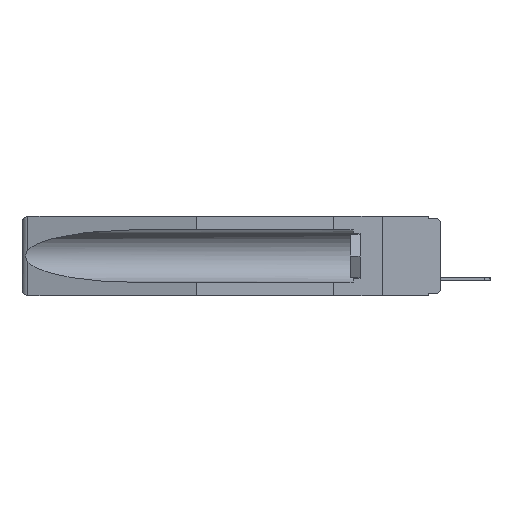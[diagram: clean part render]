
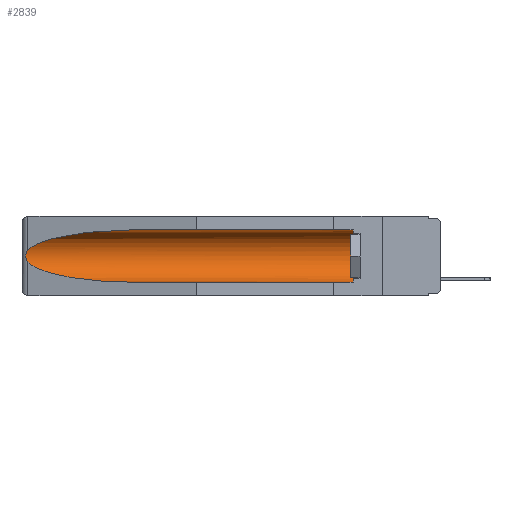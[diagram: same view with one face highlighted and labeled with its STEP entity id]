
A CAD part, left-side view. The second image highlights one B-rep face of the part: STEP entity #2839.
In plain terms, the highlighted cylindrical face has radius 2.857 mm (diameter 5.715 mm), a partial arc.
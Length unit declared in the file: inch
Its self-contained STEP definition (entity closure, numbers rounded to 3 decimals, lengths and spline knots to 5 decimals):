
#950 = CARTESIAN_POINT ( 'NONE',  ( 0.26537, 1.52718, -0.19328 ) ) ;
#1172 = DIRECTION ( 'NONE',  ( 0., 0., 1. ) ) ;
#1222 = CARTESIAN_POINT ( 'NONE',  ( 0.155, 0.126, -0.059 ) ) ;
#1223 = VERTEX_POINT ( 'NONE', #7573 ) ;
#1443 = CARTESIAN_POINT ( 'NONE',  ( 0.21114, 1.30732, -0.059 ) ) ;
#2048 = DIRECTION ( 'NONE',  ( 0., 1., 0. ) ) ;
#2408 = CARTESIAN_POINT ( 'NONE',  ( 0.21114, 1.30732, -0.284 ) ) ;
#2552 = CARTESIAN_POINT ( 'NONE',  ( 0.25451, 1.48313, -0.24835 ) ) ;
#2839 = ADVANCED_FACE ( 'NONE', ( #8455 ), #10889, .F. ) ;
#3240 = CARTESIAN_POINT ( 'NONE',  ( 0.26537, 1.52718, -0.14972 ) ) ;
#3303 = CARTESIAN_POINT ( 'NONE',  ( 0.155, 1.07973, -0.059 ) ) ;
#3367 = CIRCLE ( 'NONE', #21112, 0.1125 ) ;
#3455 = ORIENTED_EDGE ( 'NONE', *, *, #9971, .F. ) ;
#3462 =( BOUNDED_CURVE ( )  B_SPLINE_CURVE ( 3, ( #3303, #1443, #12286, #3732 ),
 .UNSPECIFIED., .F., .T. ) 
 B_SPLINE_CURVE_WITH_KNOTS ( ( 4, 4 ),
 ( 4.71239, 6.08839 ),
 .UNSPECIFIED. ) 
 CURVE ( )  GEOMETRIC_REPRESENTATION_ITEM ( )  RATIONAL_B_SPLINE_CURVE ( ( 1., 0.848, 0.848, 1. ) ) 
 REPRESENTATION_ITEM ( '' )  );
#3666 = CARTESIAN_POINT ( 'NONE',  ( 0.26655, 1.53094, -0.18657 ) ) ;
#3732 = CARTESIAN_POINT ( 'NONE',  ( 0.26537, 1.52718, -0.14972 ) ) ;
#3931 = CARTESIAN_POINT ( 'NONE',  ( 0.155, -0.30754, -0.284 ) ) ;
#5102 = VERTEX_POINT ( 'NONE', #9609 ) ;
#5926 = CARTESIAN_POINT ( 'NONE',  ( 0.26537, 1.52718, -0.19328 ) ) ;
#7573 = CARTESIAN_POINT ( 'NONE',  ( 0.26537, 1.52718, -0.14972 ) ) ;
#7783 = CARTESIAN_POINT ( 'NONE',  ( 0.26597, 1.52961, -0.15275 ) ) ;
#7817 = AXIS2_PLACEMENT_3D ( 'NONE', #23853, #2048, #15304 ) ;
#7864 = EDGE_LOOP ( 'NONE', ( #19858, #25886, #27176, #3455, #19337, #19381 ) ) ;
#8070 = CARTESIAN_POINT ( 'NONE',  ( 0.2673, 1.53269, -0.17917 ) ) ;
#8455 = FACE_OUTER_BOUND ( 'NONE', #7864, .T. ) ;
#8462 = EDGE_CURVE ( 'NONE', #27442, #5102, #19109, .T. ) ;
#8903 = DIRECTION ( 'NONE',  ( 0., 1., 0. ) ) ;
#9234 = DIRECTION ( 'NONE',  ( 0., 1., 0. ) ) ;
#9609 = CARTESIAN_POINT ( 'NONE',  ( 0.155, 1.07973, -0.284 ) ) ;
#9971 = EDGE_CURVE ( 'NONE', #14930, #5102, #11038, .T. ) ;
#10151 = DIRECTION ( 'NONE',  ( 0., -1., 0. ) ) ;
#10684 = CARTESIAN_POINT ( 'NONE',  ( 0.155, 1.07973, -0.284 ) ) ;
#10889 = CYLINDRICAL_SURFACE ( 'NONE', #7817, 0.1125 ) ;
#10970 = CARTESIAN_POINT ( 'NONE',  ( 0.155, 1.07973, -0.059 ) ) ;
#11038 = LINE ( 'NONE', #3931, #23535 ) ;
#11917 = EDGE_CURVE ( 'NONE', #17599, #1223, #3462, .T. ) ;
#12286 = CARTESIAN_POINT ( 'NONE',  ( 0.25451, 1.48313, -0.09465 ) ) ;
#14084 = CARTESIAN_POINT ( 'NONE',  ( 0.155, -0.30754, -0.059 ) ) ;
#14504 = CARTESIAN_POINT ( 'NONE',  ( 0.2673, 1.5327, -0.16383 ) ) ;
#14930 = VERTEX_POINT ( 'NONE', #25189 ) ;
#15043 = EDGE_CURVE ( 'NONE', #1223, #27442, #26823, .T. ) ;
#15304 = DIRECTION ( 'NONE',  ( 0., 0., 1. ) ) ;
#16627 = CARTESIAN_POINT ( 'NONE',  ( 0.2675, 1.53308, -0.16763 ) ) ;
#17384 = CARTESIAN_POINT ( 'NONE',  ( 0.26537, 1.52718, -0.19328 ) ) ;
#17599 = VERTEX_POINT ( 'NONE', #10970 ) ;
#18572 = CARTESIAN_POINT ( 'NONE',  ( 0.155, 0.126, -0.1715 ) ) ;
#18770 = CARTESIAN_POINT ( 'NONE',  ( 0.26654, 1.53092, -0.15636 ) ) ;
#19109 =( BOUNDED_CURVE ( )  B_SPLINE_CURVE ( 3, ( #17384, #2552, #2408, #10684 ),
 .UNSPECIFIED., .F., .T. ) 
 B_SPLINE_CURVE_WITH_KNOTS ( ( 4, 4 ),
 ( 0.1948, 1.5708 ),
 .UNSPECIFIED. ) 
 CURVE ( )  GEOMETRIC_REPRESENTATION_ITEM ( )  RATIONAL_B_SPLINE_CURVE ( ( 1., 0.848, 0.848, 1. ) ) 
 REPRESENTATION_ITEM ( '' )  );
#19337 = ORIENTED_EDGE ( 'NONE', *, *, #21934, .T. ) ;
#19381 = ORIENTED_EDGE ( 'NONE', *, *, #19422, .T. ) ;
#19422 = EDGE_CURVE ( 'NONE', #27395, #17599, #22344, .T. ) ;
#19858 = ORIENTED_EDGE ( 'NONE', *, *, #11917, .T. ) ;
#21043 = CARTESIAN_POINT ( 'NONE',  ( 0.2675, 1.53308, -0.17534 ) ) ;
#21112 = AXIS2_PLACEMENT_3D ( 'NONE', #18572, #10151, #1172 ) ;
#21934 = EDGE_CURVE ( 'NONE', #14930, #27395, #3367, .T. ) ;
#22344 = LINE ( 'NONE', #14084, #26576 ) ;
#23535 = VECTOR ( 'NONE', #8903, 39.37008 ) ;
#23853 = CARTESIAN_POINT ( 'NONE',  ( 0.155, -0.30754, -0.1715 ) ) ;
#25057 = CARTESIAN_POINT ( 'NONE',  ( 0.26597, 1.5296, -0.19026 ) ) ;
#25189 = CARTESIAN_POINT ( 'NONE',  ( 0.155, 0.126, -0.284 ) ) ;
#25886 = ORIENTED_EDGE ( 'NONE', *, *, #15043, .T. ) ;
#26576 = VECTOR ( 'NONE', #9234, 39.37008 ) ;
#26823 = B_SPLINE_CURVE_WITH_KNOTS ( 'NONE', 3,
 ( #3240, #7783, #18770, #14504, #16627, #21043, #8070, #3666, #25057, #5926 ),
 .UNSPECIFIED., .F., .F.,
 ( 4, 2, 2, 2, 4 ),
 ( 0., 0.00029, 0.00058, 0.00087, 0.00117 ),
 .UNSPECIFIED. ) ;
#27176 = ORIENTED_EDGE ( 'NONE', *, *, #8462, .T. ) ;
#27395 = VERTEX_POINT ( 'NONE', #1222 ) ;
#27442 = VERTEX_POINT ( 'NONE', #950 ) ;
